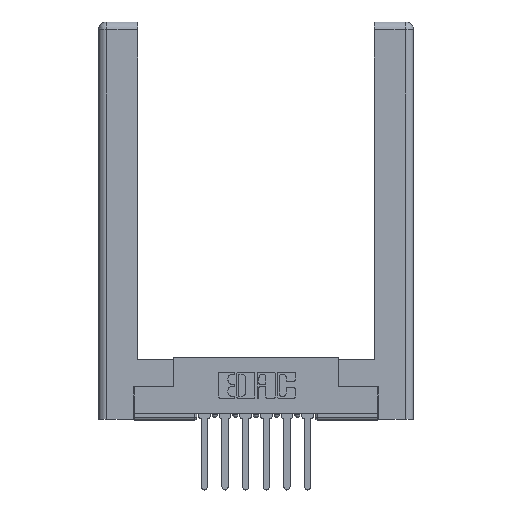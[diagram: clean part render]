
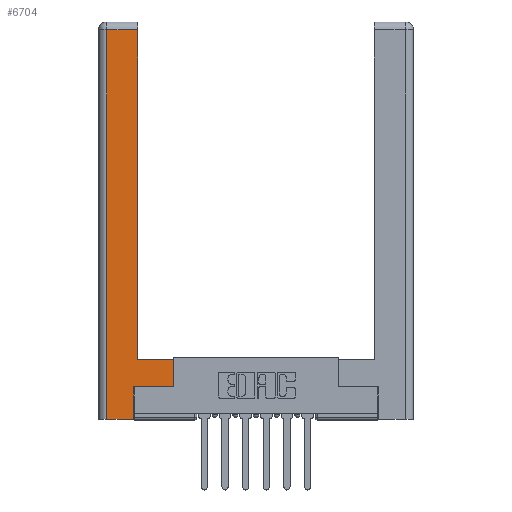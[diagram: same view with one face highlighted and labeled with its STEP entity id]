
A CAD part, top view. The second image highlights one B-rep face of the part: STEP entity #6704.
In plain terms, the highlighted planar face has unit normal (0, 0, 1).
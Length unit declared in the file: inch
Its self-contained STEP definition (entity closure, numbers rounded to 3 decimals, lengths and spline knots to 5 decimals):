
#508 = CARTESIAN_POINT ( 'NONE',  ( 0.565, 0.245, 0. ) ) ;
#682 = CARTESIAN_POINT ( 'NONE',  ( 0.0615, 2.94, 0. ) ) ;
#718 = ORIENTED_EDGE ( 'NONE', *, *, #7935, .T. ) ;
#1086 = VECTOR ( 'NONE', #8403, 39.37008 ) ;
#1117 = CARTESIAN_POINT ( 'NONE',  ( 0.565, 0.245, 0. ) ) ;
#1351 = EDGE_CURVE ( 'NONE', #2225, #11914, #4423, .T. ) ;
#1561 = CARTESIAN_POINT ( 'NONE',  ( 0.295, 2.94, 0. ) ) ;
#1605 = CARTESIAN_POINT ( 'NONE',  ( 0.265, 0.245, 0. ) ) ;
#1760 = VERTEX_POINT ( 'NONE', #508 ) ;
#2225 = VERTEX_POINT ( 'NONE', #1561 ) ;
#2341 = CARTESIAN_POINT ( 'NONE',  ( 0.565, 0.45, 0. ) ) ;
#2379 = LINE ( 'NONE', #3203, #3172 ) ;
#2720 = LINE ( 'NONE', #6426, #7140 ) ;
#3054 = VECTOR ( 'NONE', #11005, 39.37008 ) ;
#3071 = PLANE ( 'NONE',  #9898 ) ;
#3172 = VECTOR ( 'NONE', #8073, 39.37008 ) ;
#3203 = CARTESIAN_POINT ( 'NONE',  ( 0.295, 0.45, 0. ) ) ;
#3459 = CARTESIAN_POINT ( 'NONE',  ( 0.565, 0.45, 0. ) ) ;
#3889 = DIRECTION ( 'NONE',  ( 0., 0., -1. ) ) ;
#3948 = CARTESIAN_POINT ( 'NONE',  ( 0., 0., 0. ) ) ;
#4043 = ORIENTED_EDGE ( 'NONE', *, *, #5964, .T. ) ;
#4078 = VECTOR ( 'NONE', #7336, 39.37008 ) ;
#4098 = CARTESIAN_POINT ( 'NONE',  ( 0.265, 0., 0. ) ) ;
#4177 = LINE ( 'NONE', #7916, #10179 ) ;
#4217 = CARTESIAN_POINT ( 'NONE',  ( 0.265, 0.245, 0. ) ) ;
#4423 = LINE ( 'NONE', #10189, #3054 ) ;
#4826 = DIRECTION ( 'NONE',  ( 1., 0., 0. ) ) ;
#5049 = VERTEX_POINT ( 'NONE', #3459 ) ;
#5717 = ORIENTED_EDGE ( 'NONE', *, *, #7048, .T. ) ;
#5841 = VERTEX_POINT ( 'NONE', #4098 ) ;
#5964 = EDGE_CURVE ( 'NONE', #5841, #6251, #8170, .T. ) ;
#6067 = ORIENTED_EDGE ( 'NONE', *, *, #12285, .T. ) ;
#6231 = ORIENTED_EDGE ( 'NONE', *, *, #1351, .T. ) ;
#6251 = VERTEX_POINT ( 'NONE', #4217 ) ;
#6426 = CARTESIAN_POINT ( 'NONE',  ( 0.0615, 0., 0. ) ) ;
#6520 = CARTESIAN_POINT ( 'NONE',  ( 0.295, 0.45, 0. ) ) ;
#6556 = VERTEX_POINT ( 'NONE', #6639 ) ;
#6639 = CARTESIAN_POINT ( 'NONE',  ( 0.0615, 0., 0. ) ) ;
#6704 = ADVANCED_FACE ( 'NONE', ( #10796 ), #3071, .F. ) ;
#7048 = EDGE_CURVE ( 'NONE', #6556, #5841, #7382, .T. ) ;
#7084 = DIRECTION ( 'NONE',  ( 0., 1., 0. ) ) ;
#7140 = VECTOR ( 'NONE', #9439, 39.37008 ) ;
#7335 = VECTOR ( 'NONE', #4826, 39.37008 ) ;
#7336 = DIRECTION ( 'NONE',  ( 0., 1., 0. ) ) ;
#7382 = LINE ( 'NONE', #10411, #1086 ) ;
#7916 = CARTESIAN_POINT ( 'NONE',  ( 0.295, 3., 0. ) ) ;
#7935 = EDGE_CURVE ( 'NONE', #5049, #10791, #2379, .T. ) ;
#8073 = DIRECTION ( 'NONE',  ( -1., 0., 0. ) ) ;
#8170 = LINE ( 'NONE', #1605, #4078 ) ;
#8391 = EDGE_LOOP ( 'NONE', ( #12248, #6231, #6067, #5717, #4043, #10365, #10691, #718 ) ) ;
#8403 = DIRECTION ( 'NONE',  ( 1., 0., 0. ) ) ;
#8933 = EDGE_CURVE ( 'NONE', #1760, #5049, #11122, .T. ) ;
#9439 = DIRECTION ( 'NONE',  ( 0., -1., 0. ) ) ;
#9898 = AXIS2_PLACEMENT_3D ( 'NONE', #3948, #3889, #11601 ) ;
#10179 = VECTOR ( 'NONE', #11950, 39.37008 ) ;
#10189 = CARTESIAN_POINT ( 'NONE',  ( 0.0615, 2.94, 0. ) ) ;
#10365 = ORIENTED_EDGE ( 'NONE', *, *, #11635, .T. ) ;
#10411 = CARTESIAN_POINT ( 'NONE',  ( 0.265, 0., 0. ) ) ;
#10545 = VECTOR ( 'NONE', #7084, 39.37008 ) ;
#10603 = LINE ( 'NONE', #1117, #7335 ) ;
#10691 = ORIENTED_EDGE ( 'NONE', *, *, #8933, .T. ) ;
#10791 = VERTEX_POINT ( 'NONE', #6520 ) ;
#10796 = FACE_OUTER_BOUND ( 'NONE', #8391, .T. ) ;
#11005 = DIRECTION ( 'NONE',  ( -1., 0., 0. ) ) ;
#11122 = LINE ( 'NONE', #2341, #10545 ) ;
#11601 = DIRECTION ( 'NONE',  ( -1., 0., 0. ) ) ;
#11635 = EDGE_CURVE ( 'NONE', #6251, #1760, #10603, .T. ) ;
#11914 = VERTEX_POINT ( 'NONE', #682 ) ;
#11950 = DIRECTION ( 'NONE',  ( 0., 1., 0. ) ) ;
#12113 = EDGE_CURVE ( 'NONE', #10791, #2225, #4177, .T. ) ;
#12248 = ORIENTED_EDGE ( 'NONE', *, *, #12113, .T. ) ;
#12285 = EDGE_CURVE ( 'NONE', #11914, #6556, #2720, .T. ) ;
